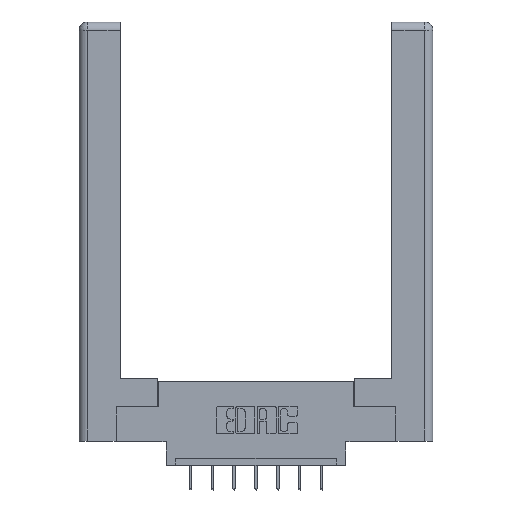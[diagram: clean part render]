
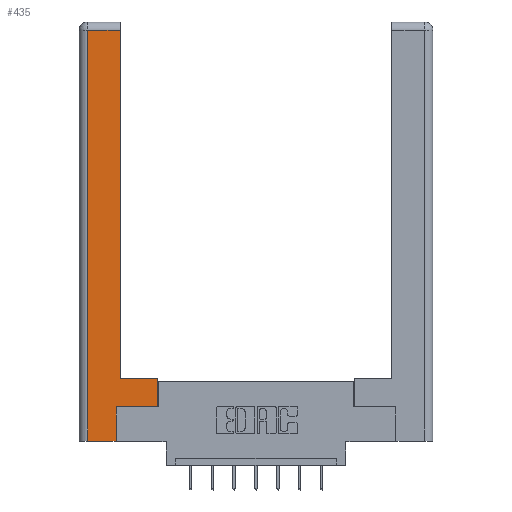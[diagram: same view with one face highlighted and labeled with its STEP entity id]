
A CAD part, top view. The second image highlights one B-rep face of the part: STEP entity #435.
In plain terms, the highlighted planar face has unit normal (0, 0, 1).
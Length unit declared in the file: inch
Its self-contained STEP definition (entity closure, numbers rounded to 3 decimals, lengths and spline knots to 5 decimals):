
#183 = ORIENTED_EDGE ( 'NONE', *, *, #5001, .T. ) ;
#435 = ADVANCED_FACE ( 'NONE', ( #6190 ), #7550, .F. ) ;
#503 = ORIENTED_EDGE ( 'NONE', *, *, #11637, .T. ) ;
#527 = CARTESIAN_POINT ( 'NONE',  ( 0.0615, 2.94, 0. ) ) ;
#1177 = CARTESIAN_POINT ( 'NONE',  ( 0.265, 0.245, 0. ) ) ;
#1200 = EDGE_CURVE ( 'NONE', #6638, #9850, #10254, .T. ) ;
#1299 = EDGE_CURVE ( 'NONE', #6648, #10749, #9027, .T. ) ;
#1362 = VERTEX_POINT ( 'NONE', #11775 ) ;
#1466 = LINE ( 'NONE', #2872, #5120 ) ;
#1735 = CARTESIAN_POINT ( 'NONE',  ( 0., 0., 0. ) ) ;
#1860 = DIRECTION ( 'NONE',  ( -1., 0., 0. ) ) ;
#2091 = CARTESIAN_POINT ( 'NONE',  ( 0.295, 2.94, 0. ) ) ;
#2170 = CARTESIAN_POINT ( 'NONE',  ( 0.295, 3., 0. ) ) ;
#2172 = ORIENTED_EDGE ( 'NONE', *, *, #5856, .T. ) ;
#2335 = VECTOR ( 'NONE', #9111, 39.37008 ) ;
#2472 = VECTOR ( 'NONE', #3880, 39.37008 ) ;
#2512 = LINE ( 'NONE', #5053, #7826 ) ;
#2872 = CARTESIAN_POINT ( 'NONE',  ( 0.565, 0.45, 0. ) ) ;
#3514 = CARTESIAN_POINT ( 'NONE',  ( 0.0615, 0., 0. ) ) ;
#3633 = CARTESIAN_POINT ( 'NONE',  ( 0.0615, 0., 0. ) ) ;
#3826 = EDGE_CURVE ( 'NONE', #7025, #1362, #10034, .T. ) ;
#3880 = DIRECTION ( 'NONE',  ( 0., 1., 0. ) ) ;
#4425 = ORIENTED_EDGE ( 'NONE', *, *, #5903, .T. ) ;
#5001 = EDGE_CURVE ( 'NONE', #7615, #7025, #1466, .T. ) ;
#5053 = CARTESIAN_POINT ( 'NONE',  ( 0.265, 0., 0. ) ) ;
#5095 = DIRECTION ( 'NONE',  ( 1., 0., 0. ) ) ;
#5120 = VECTOR ( 'NONE', #11693, 39.37008 ) ;
#5235 = ORIENTED_EDGE ( 'NONE', *, *, #12196, .T. ) ;
#5406 = CARTESIAN_POINT ( 'NONE',  ( 0.0615, 2.94, 0. ) ) ;
#5582 = DIRECTION ( 'NONE',  ( 0., -1., 0. ) ) ;
#5856 = EDGE_CURVE ( 'NONE', #10749, #6638, #2512, .T. ) ;
#5903 = EDGE_CURVE ( 'NONE', #12524, #6648, #7686, .T. ) ;
#6190 = FACE_OUTER_BOUND ( 'NONE', #7947, .T. ) ;
#6436 = LINE ( 'NONE', #2170, #2335 ) ;
#6588 = VECTOR ( 'NONE', #5582, 39.37008 ) ;
#6638 = VERTEX_POINT ( 'NONE', #8124 ) ;
#6648 = VERTEX_POINT ( 'NONE', #527 ) ;
#7025 = VERTEX_POINT ( 'NONE', #9779 ) ;
#7348 = DIRECTION ( 'NONE',  ( -1., 0., 0. ) ) ;
#7550 = PLANE ( 'NONE',  #12127 ) ;
#7615 = VERTEX_POINT ( 'NONE', #9308 ) ;
#7681 = DIRECTION ( 'NONE',  ( 0., 0., -1. ) ) ;
#7686 = LINE ( 'NONE', #5406, #9685 ) ;
#7826 = VECTOR ( 'NONE', #5095, 39.37008 ) ;
#7947 = EDGE_LOOP ( 'NONE', ( #503, #4425, #10800, #2172, #11168, #5235, #183, #10751 ) ) ;
#8032 = VECTOR ( 'NONE', #8820, 39.37008 ) ;
#8124 = CARTESIAN_POINT ( 'NONE',  ( 0.265, 0., 0. ) ) ;
#8707 = VECTOR ( 'NONE', #10889, 39.37008 ) ;
#8820 = DIRECTION ( 'NONE',  ( -1., 0., 0. ) ) ;
#8883 = LINE ( 'NONE', #11590, #8707 ) ;
#9027 = LINE ( 'NONE', #3633, #6588 ) ;
#9111 = DIRECTION ( 'NONE',  ( 0., 1., 0. ) ) ;
#9308 = CARTESIAN_POINT ( 'NONE',  ( 0.565, 0.245, 0. ) ) ;
#9685 = VECTOR ( 'NONE', #7348, 39.37008 ) ;
#9779 = CARTESIAN_POINT ( 'NONE',  ( 0.565, 0.45, 0. ) ) ;
#9788 = CARTESIAN_POINT ( 'NONE',  ( 0.265, 0.245, 0. ) ) ;
#9850 = VERTEX_POINT ( 'NONE', #1177 ) ;
#10034 = LINE ( 'NONE', #10654, #8032 ) ;
#10254 = LINE ( 'NONE', #9788, #2472 ) ;
#10654 = CARTESIAN_POINT ( 'NONE',  ( 0.295, 0.45, 0. ) ) ;
#10749 = VERTEX_POINT ( 'NONE', #3514 ) ;
#10751 = ORIENTED_EDGE ( 'NONE', *, *, #3826, .T. ) ;
#10800 = ORIENTED_EDGE ( 'NONE', *, *, #1299, .T. ) ;
#10889 = DIRECTION ( 'NONE',  ( 1., 0., 0. ) ) ;
#11168 = ORIENTED_EDGE ( 'NONE', *, *, #1200, .T. ) ;
#11590 = CARTESIAN_POINT ( 'NONE',  ( 0.565, 0.245, 0. ) ) ;
#11637 = EDGE_CURVE ( 'NONE', #1362, #12524, #6436, .T. ) ;
#11693 = DIRECTION ( 'NONE',  ( 0., 1., 0. ) ) ;
#11775 = CARTESIAN_POINT ( 'NONE',  ( 0.295, 0.45, 0. ) ) ;
#12127 = AXIS2_PLACEMENT_3D ( 'NONE', #1735, #7681, #1860 ) ;
#12196 = EDGE_CURVE ( 'NONE', #9850, #7615, #8883, .T. ) ;
#12524 = VERTEX_POINT ( 'NONE', #2091 ) ;
